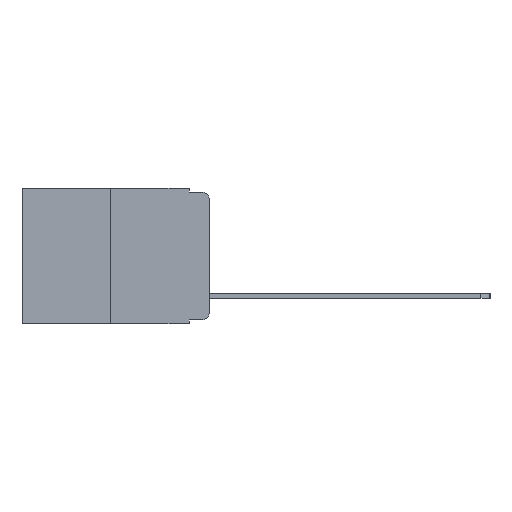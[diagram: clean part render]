
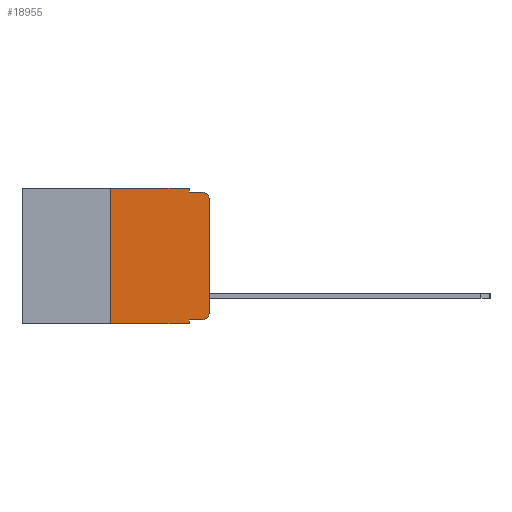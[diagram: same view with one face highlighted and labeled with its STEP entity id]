
A CAD part, left-side view. The second image highlights one B-rep face of the part: STEP entity #18955.
In plain terms, the highlighted planar face has unit normal (-1, 0, 0).
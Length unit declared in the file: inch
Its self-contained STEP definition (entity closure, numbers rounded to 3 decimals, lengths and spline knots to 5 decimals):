
#160 = EDGE_CURVE ( 'NONE', #18477, #8566, #11570, .T. ) ;
#280 = ORIENTED_EDGE ( 'NONE', *, *, #5125, .F. ) ;
#406 = CARTESIAN_POINT ( 'NONE',  ( 0., 0.02, -0.333 ) ) ;
#607 = VERTEX_POINT ( 'NONE', #9942 ) ;
#866 = EDGE_CURVE ( 'NONE', #18477, #14406, #11731, .T. ) ;
#1052 = CARTESIAN_POINT ( 'NONE',  ( 0., 0.051, 0. ) ) ;
#1264 = LINE ( 'NONE', #17037, #12583 ) ;
#1383 = AXIS2_PLACEMENT_3D ( 'NONE', #10660, #1417, #12183 ) ;
#1417 = DIRECTION ( 'NONE',  ( 1., 0., 0. ) ) ;
#1876 = CARTESIAN_POINT ( 'NONE',  ( 0., 0.25, 0. ) ) ;
#2430 = ORIENTED_EDGE ( 'NONE', *, *, #866, .F. ) ;
#2469 = CARTESIAN_POINT ( 'NONE',  ( 0., 0.051, -0.343 ) ) ;
#2701 = ORIENTED_EDGE ( 'NONE', *, *, #4348, .T. ) ;
#2775 = EDGE_CURVE ( 'NONE', #11645, #14406, #1264, .T. ) ;
#2885 = DIRECTION ( 'NONE',  ( -1., 0., 0. ) ) ;
#3024 = CARTESIAN_POINT ( 'NONE',  ( 0., 0.051, -0.333 ) ) ;
#3067 = EDGE_CURVE ( 'NONE', #11645, #18153, #15687, .T. ) ;
#3343 = EDGE_CURVE ( 'NONE', #13874, #10820, #3532, .T. ) ;
#3375 = ORIENTED_EDGE ( 'NONE', *, *, #2775, .T. ) ;
#3520 = ORIENTED_EDGE ( 'NONE', *, *, #14686, .T. ) ;
#3532 = LINE ( 'NONE', #10385, #10664 ) ;
#3780 = VECTOR ( 'NONE', #16546, 39.37008 ) ;
#3922 = LINE ( 'NONE', #1052, #19023 ) ;
#4144 = DIRECTION ( 'NONE',  ( 0., 0., -1. ) ) ;
#4348 = EDGE_CURVE ( 'NONE', #18399, #10820, #12760, .T. ) ;
#4532 = CARTESIAN_POINT ( 'NONE',  ( 0., 0.051, -0.01 ) ) ;
#4600 = CARTESIAN_POINT ( 'NONE',  ( 0., 0.473, 0. ) ) ;
#4780 = DIRECTION ( 'NONE',  ( 0., 0., -1. ) ) ;
#4846 = ORIENTED_EDGE ( 'NONE', *, *, #3067, .F. ) ;
#5125 = EDGE_CURVE ( 'NONE', #607, #13874, #3922, .T. ) ;
#5207 = EDGE_LOOP ( 'NONE', ( #3520, #2701, #19316, #280, #17384, #4846, #3375, #2430, #10995, #15389 ) ) ;
#5842 = CARTESIAN_POINT ( 'NONE',  ( 0., 0.25, -0.343 ) ) ;
#5911 = DIRECTION ( 'NONE',  ( 0., -1., 0. ) ) ;
#6809 = CARTESIAN_POINT ( 'NONE',  ( 0., 0., -0.313 ) ) ;
#7349 = DIRECTION ( 'NONE',  ( 0., 0., -1. ) ) ;
#8566 = VERTEX_POINT ( 'NONE', #406 ) ;
#8944 = EDGE_CURVE ( 'NONE', #18153, #607, #14959, .T. ) ;
#9230 = DIRECTION ( 'NONE',  ( 0., -1., 0. ) ) ;
#9942 = CARTESIAN_POINT ( 'NONE',  ( 0., 0.051, 0. ) ) ;
#10206 = CIRCLE ( 'NONE', #16532, 0.02 ) ;
#10316 = DIRECTION ( 'NONE',  ( 0., -1., 0. ) ) ;
#10385 = CARTESIAN_POINT ( 'NONE',  ( 0., 0.051, -0.01 ) ) ;
#10660 = CARTESIAN_POINT ( 'NONE',  ( 0., 0.473, 0. ) ) ;
#10664 = VECTOR ( 'NONE', #10316, 39.37008 ) ;
#10820 = VERTEX_POINT ( 'NONE', #11355 ) ;
#10851 = VECTOR ( 'NONE', #19307, 39.37008 ) ;
#10995 = ORIENTED_EDGE ( 'NONE', *, *, #160, .T. ) ;
#11103 = CARTESIAN_POINT ( 'NONE',  ( 0., 0.02, -0.03 ) ) ;
#11260 = VECTOR ( 'NONE', #4144, 39.37008 ) ;
#11355 = CARTESIAN_POINT ( 'NONE',  ( 0., 0.02, -0.01 ) ) ;
#11570 = LINE ( 'NONE', #3024, #18195 ) ;
#11645 = VERTEX_POINT ( 'NONE', #5842 ) ;
#11731 = LINE ( 'NONE', #14376, #11260 ) ;
#12024 = CARTESIAN_POINT ( 'NONE',  ( 0., 0.02, -0.313 ) ) ;
#12183 = DIRECTION ( 'NONE',  ( 0., 0., -1. ) ) ;
#12268 = CARTESIAN_POINT ( 'NONE',  ( 0., 0.051, -0.333 ) ) ;
#12583 = VECTOR ( 'NONE', #17091, 39.37008 ) ;
#12760 = CIRCLE ( 'NONE', #17806, 0.02 ) ;
#13103 = FACE_OUTER_BOUND ( 'NONE', #5207, .T. ) ;
#13345 = EDGE_CURVE ( 'NONE', #8566, #18281, #10206, .T. ) ;
#13507 = DIRECTION ( 'NONE',  ( 0., 0., -1. ) ) ;
#13874 = VERTEX_POINT ( 'NONE', #4532 ) ;
#13890 = DIRECTION ( 'NONE',  ( -1., 0., 0. ) ) ;
#14376 = CARTESIAN_POINT ( 'NONE',  ( 0., 0.051, 0. ) ) ;
#14406 = VERTEX_POINT ( 'NONE', #2469 ) ;
#14686 = EDGE_CURVE ( 'NONE', #18281, #18399, #14740, .T. ) ;
#14740 = LINE ( 'NONE', #15168, #10851 ) ;
#14959 = LINE ( 'NONE', #4600, #18180 ) ;
#15168 = CARTESIAN_POINT ( 'NONE',  ( 0., 0., 0. ) ) ;
#15389 = ORIENTED_EDGE ( 'NONE', *, *, #13345, .T. ) ;
#15687 = LINE ( 'NONE', #17668, #3780 ) ;
#16380 = PLANE ( 'NONE',  #1383 ) ;
#16398 = CARTESIAN_POINT ( 'NONE',  ( 0., 0., -0.03 ) ) ;
#16532 = AXIS2_PLACEMENT_3D ( 'NONE', #12024, #2885, #13507 ) ;
#16546 = DIRECTION ( 'NONE',  ( 0., 0., 1. ) ) ;
#17037 = CARTESIAN_POINT ( 'NONE',  ( 0., 0.473, -0.343 ) ) ;
#17091 = DIRECTION ( 'NONE',  ( 0., -1., 0. ) ) ;
#17384 = ORIENTED_EDGE ( 'NONE', *, *, #8944, .F. ) ;
#17668 = CARTESIAN_POINT ( 'NONE',  ( 0., 0.25, 0. ) ) ;
#17806 = AXIS2_PLACEMENT_3D ( 'NONE', #11103, #13890, #4780 ) ;
#18153 = VERTEX_POINT ( 'NONE', #1876 ) ;
#18180 = VECTOR ( 'NONE', #9230, 39.37008 ) ;
#18195 = VECTOR ( 'NONE', #5911, 39.37008 ) ;
#18281 = VERTEX_POINT ( 'NONE', #6809 ) ;
#18399 = VERTEX_POINT ( 'NONE', #16398 ) ;
#18477 = VERTEX_POINT ( 'NONE', #12268 ) ;
#18955 = ADVANCED_FACE ( 'NONE', ( #13103 ), #16380, .F. ) ;
#19023 = VECTOR ( 'NONE', #7349, 39.37008 ) ;
#19307 = DIRECTION ( 'NONE',  ( 0., 0., 1. ) ) ;
#19316 = ORIENTED_EDGE ( 'NONE', *, *, #3343, .F. ) ;
